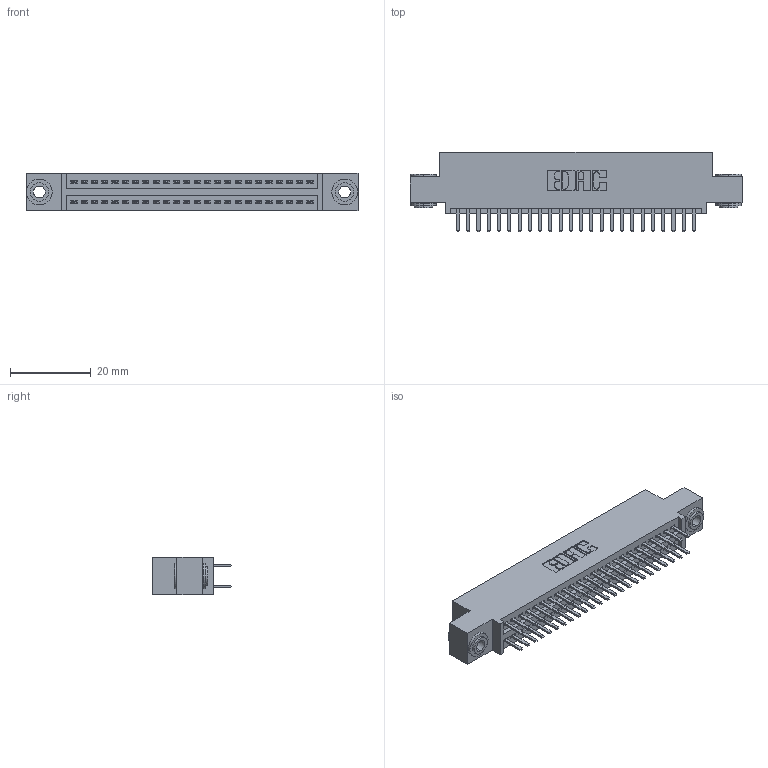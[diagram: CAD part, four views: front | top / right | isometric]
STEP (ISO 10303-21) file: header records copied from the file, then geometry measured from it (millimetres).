
FILE_DESCRIPTION (( 'STEP AP203' ), '1' );
FILE_NAME ('345-048-520-503.STEP', '2018-09-11T10:00:50', ( '' ), ( '' ), 'SwSTEP 2.0', 'SolidWorks 2016', '' );
FILE_SCHEMA (( 'CONFIG_CONTROL_DESIGN' ));
Length unit declared in the file: inch
Products named in the file (4): 345 Part_0.110 Offset - 0.156 Dia-TH; 345-292-001_345-293-120; 345-250-002_345-250-002-102; 345-048-520-503
Assembly tree (51 placements, depth 2):
  345-048-520-503
    345 Part_0.110 Offset - 0.156 Dia-TH
    345-292-001_345-293-120  x48
    345-250-002_345-250-002-102  x2
Bounding box: 82.17 x 19.68 x 9.4 mm (x, y, z)
Volume: 7739.8 mm3; surface area: 11345 mm2
Topology: 51 solids, 51 shells, 2760 faces, 7965 edges, 5178 vertices
Faces by surface type: plane 1774, cylinder 978, cone 8
Entity records: 22150 total; most frequent: CARTESIAN_POINT 3719, ORIENTED_EDGE 3634, DIRECTION 3319, EDGE_CURVE 1817, LINE 1561, VECTOR 1561, VERTEX_POINT 1206, AXIS2_PLACEMENT_3D 879
